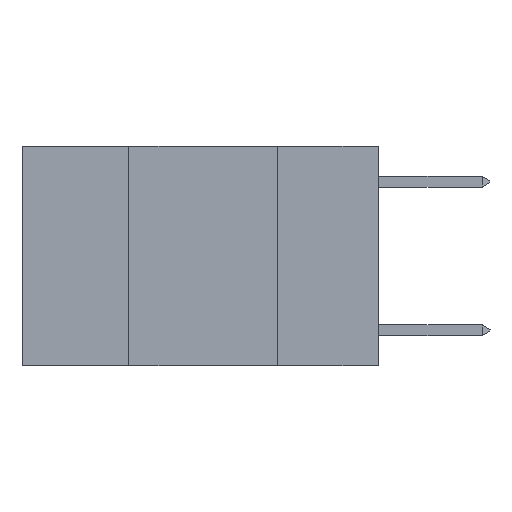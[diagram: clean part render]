
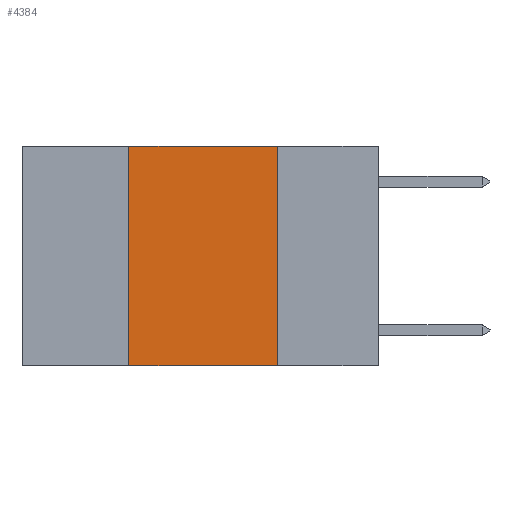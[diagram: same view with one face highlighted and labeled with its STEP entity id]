
A CAD part, left-side view. The second image highlights one B-rep face of the part: STEP entity #4384.
In plain terms, the highlighted planar face has unit normal (-1, 0, 0).
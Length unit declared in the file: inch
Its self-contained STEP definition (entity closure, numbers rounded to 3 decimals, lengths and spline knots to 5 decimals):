
#388 = DIRECTION ( 'NONE',  ( 0., 0., -1. ) ) ;
#888 = VERTEX_POINT ( 'NONE', #4794 ) ;
#968 = EDGE_CURVE ( 'NONE', #888, #4982, #5296, .T. ) ;
#1199 = LINE ( 'NONE', #7393, #8399 ) ;
#1274 = DIRECTION ( 'NONE',  ( 0., 0., -1. ) ) ;
#1551 = CARTESIAN_POINT ( 'NONE',  ( 0., 0.42, -0.37 ) ) ;
#1663 = DIRECTION ( 'NONE',  ( 0., 0., 1. ) ) ;
#1809 = VECTOR ( 'NONE', #3569, 39.37008 ) ;
#2561 = AXIS2_PLACEMENT_3D ( 'NONE', #4053, #5465, #1274 ) ;
#3002 = CARTESIAN_POINT ( 'NONE',  ( 0., 0.6, 0. ) ) ;
#3569 = DIRECTION ( 'NONE',  ( 0., -1., 0. ) ) ;
#3894 = LINE ( 'NONE', #7091, #1809 ) ;
#4053 = CARTESIAN_POINT ( 'NONE',  ( 0., 0.6, 0. ) ) ;
#4384 = ADVANCED_FACE ( 'NONE', ( #7666 ), #6155, .F. ) ;
#4430 = DIRECTION ( 'NONE',  ( 0., -1., 0. ) ) ;
#4687 = VERTEX_POINT ( 'NONE', #7856 ) ;
#4779 = EDGE_CURVE ( 'NONE', #6171, #888, #4815, .T. ) ;
#4794 = CARTESIAN_POINT ( 'NONE',  ( 0., 0.42, 0. ) ) ;
#4815 = LINE ( 'NONE', #7247, #6449 ) ;
#4982 = VERTEX_POINT ( 'NONE', #5401 ) ;
#5296 = LINE ( 'NONE', #3002, #6954 ) ;
#5401 = CARTESIAN_POINT ( 'NONE',  ( 0., 0.17, 0. ) ) ;
#5465 = DIRECTION ( 'NONE',  ( 1., 0., 0. ) ) ;
#5705 = EDGE_CURVE ( 'NONE', #4982, #4687, #1199, .T. ) ;
#6014 = ORIENTED_EDGE ( 'NONE', *, *, #5705, .F. ) ;
#6148 = ORIENTED_EDGE ( 'NONE', *, *, #8289, .T. ) ;
#6155 = PLANE ( 'NONE',  #2561 ) ;
#6171 = VERTEX_POINT ( 'NONE', #1551 ) ;
#6331 = EDGE_LOOP ( 'NONE', ( #6014, #8465, #7000, #6148 ) ) ;
#6449 = VECTOR ( 'NONE', #1663, 39.37008 ) ;
#6954 = VECTOR ( 'NONE', #4430, 39.37008 ) ;
#7000 = ORIENTED_EDGE ( 'NONE', *, *, #4779, .F. ) ;
#7091 = CARTESIAN_POINT ( 'NONE',  ( 0., 0.6, -0.37 ) ) ;
#7247 = CARTESIAN_POINT ( 'NONE',  ( 0., 0.42, 0. ) ) ;
#7393 = CARTESIAN_POINT ( 'NONE',  ( 0., 0.17, 0. ) ) ;
#7666 = FACE_OUTER_BOUND ( 'NONE', #6331, .T. ) ;
#7856 = CARTESIAN_POINT ( 'NONE',  ( 0., 0.17, -0.37 ) ) ;
#8289 = EDGE_CURVE ( 'NONE', #6171, #4687, #3894, .T. ) ;
#8399 = VECTOR ( 'NONE', #388, 39.37008 ) ;
#8465 = ORIENTED_EDGE ( 'NONE', *, *, #968, .F. ) ;
